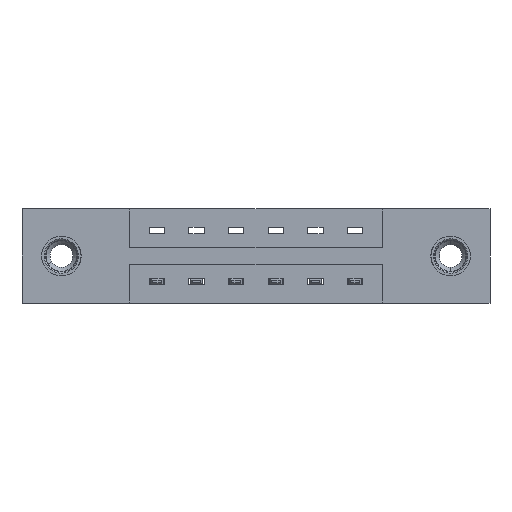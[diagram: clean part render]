
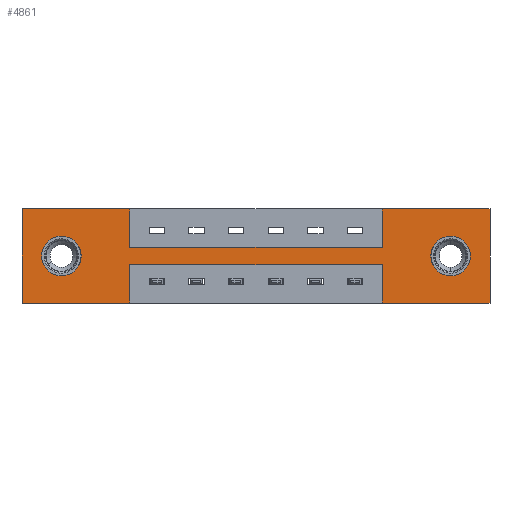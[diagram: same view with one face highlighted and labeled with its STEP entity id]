
A CAD part, front view. The second image highlights one B-rep face of the part: STEP entity #4861.
In plain terms, the highlighted planar face has unit normal (0, -1, 0).
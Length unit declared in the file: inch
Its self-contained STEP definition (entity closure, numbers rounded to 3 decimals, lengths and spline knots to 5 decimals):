
#3 = CARTESIAN_POINT ( 'NONE',  ( 1.417, 0., 0. ) ) ;
#84 = DIRECTION ( 'NONE',  ( 0., 1., 0. ) ) ;
#86 = CARTESIAN_POINT ( 'NONE',  ( 0., 0., -0.37 ) ) ;
#117 = VERTEX_POINT ( 'NONE', #8231 ) ;
#158 = EDGE_CURVE ( 'NONE', #1358, #7796, #9642, .T. ) ;
#309 = CARTESIAN_POINT ( 'NONE',  ( 0.155, 0., -0.185 ) ) ;
#356 = AXIS2_PLACEMENT_3D ( 'NONE', #9466, #7812, #4768 ) ;
#578 = ORIENTED_EDGE ( 'NONE', *, *, #1688, .F. ) ;
#599 = EDGE_LOOP ( 'NONE', ( #6540, #2924 ) ) ;
#604 = EDGE_CURVE ( 'NONE', #5155, #1770, #6991, .T. ) ;
#765 = EDGE_CURVE ( 'NONE', #10042, #5155, #3315, .T. ) ;
#847 = CARTESIAN_POINT ( 'NONE',  ( 0.425, 0., -0.22 ) ) ;
#882 = ORIENTED_EDGE ( 'NONE', *, *, #9879, .T. ) ;
#915 = VERTEX_POINT ( 'NONE', #2943 ) ;
#984 = ORIENTED_EDGE ( 'NONE', *, *, #6231, .T. ) ;
#1147 = CARTESIAN_POINT ( 'NONE',  ( 0.425, 0., 0. ) ) ;
#1316 = ORIENTED_EDGE ( 'NONE', *, *, #3263, .F. ) ;
#1358 = VERTEX_POINT ( 'NONE', #2992 ) ;
#1425 = CARTESIAN_POINT ( 'NONE',  ( 0., 0., -0.37 ) ) ;
#1584 = ORIENTED_EDGE ( 'NONE', *, *, #7878, .F. ) ;
#1679 = VECTOR ( 'NONE', #5977, 39.37008 ) ;
#1688 = EDGE_CURVE ( 'NONE', #4008, #117, #4629, .T. ) ;
#1770 = VERTEX_POINT ( 'NONE', #3680 ) ;
#1782 = VERTEX_POINT ( 'NONE', #7600 ) ;
#1876 = FACE_OUTER_BOUND ( 'NONE', #7864, .T. ) ;
#1889 = VERTEX_POINT ( 'NONE', #1425 ) ;
#1912 = CARTESIAN_POINT ( 'NONE',  ( 0., 0., 0. ) ) ;
#1924 = DIRECTION ( 'NONE',  ( 1., 0., 0. ) ) ;
#1983 = DIRECTION ( 'NONE',  ( 0., 0., -1. ) ) ;
#2023 = LINE ( 'NONE', #4361, #3880 ) ;
#2325 = PLANE ( 'NONE',  #356 ) ;
#2485 = DIRECTION ( 'NONE',  ( 0., 0., 1. ) ) ;
#2545 = VECTOR ( 'NONE', #1983, 39.37008 ) ;
#2671 = CARTESIAN_POINT ( 'NONE',  ( 1.687, 0., -0.263 ) ) ;
#2788 = CARTESIAN_POINT ( 'NONE',  ( 1.417, 0., -0.37 ) ) ;
#2924 = ORIENTED_EDGE ( 'NONE', *, *, #3849, .T. ) ;
#2937 = DIRECTION ( 'NONE',  ( 0., 0., -1. ) ) ;
#2943 = CARTESIAN_POINT ( 'NONE',  ( 0.425, 0., -0.37 ) ) ;
#2992 = CARTESIAN_POINT ( 'NONE',  ( 1.417, 0., -0.22 ) ) ;
#3064 = EDGE_CURVE ( 'NONE', #1770, #5269, #2023, .T. ) ;
#3070 = LINE ( 'NONE', #1912, #3682 ) ;
#3109 = AXIS2_PLACEMENT_3D ( 'NONE', #309, #8178, #6662 ) ;
#3122 = CIRCLE ( 'NONE', #3109, 0.078 ) ;
#3217 = AXIS2_PLACEMENT_3D ( 'NONE', #4790, #84, #6390 ) ;
#3255 = CARTESIAN_POINT ( 'NONE',  ( 0.155, 0., -0.185 ) ) ;
#3263 = EDGE_CURVE ( 'NONE', #7796, #915, #5581, .T. ) ;
#3315 = LINE ( 'NONE', #3959, #8549 ) ;
#3343 = AXIS2_PLACEMENT_3D ( 'NONE', #3255, #8640, #2485 ) ;
#3445 = CIRCLE ( 'NONE', #3989, 0.078 ) ;
#3448 = ORIENTED_EDGE ( 'NONE', *, *, #3064, .F. ) ;
#3455 = EDGE_LOOP ( 'NONE', ( #882, #984 ) ) ;
#3488 = DIRECTION ( 'NONE',  ( -1., 0., 0. ) ) ;
#3560 = VERTEX_POINT ( 'NONE', #8334 ) ;
#3680 = CARTESIAN_POINT ( 'NONE',  ( 1.417, 0., -0.15 ) ) ;
#3682 = VECTOR ( 'NONE', #9717, 39.37008 ) ;
#3849 = EDGE_CURVE ( 'NONE', #7292, #8692, #3122, .T. ) ;
#3880 = VECTOR ( 'NONE', #9771, 39.37008 ) ;
#3893 = CIRCLE ( 'NONE', #3343, 0.078 ) ;
#3951 = EDGE_CURVE ( 'NONE', #117, #5256, #4829, .T. ) ;
#3959 = CARTESIAN_POINT ( 'NONE',  ( 0.425, 0., 0. ) ) ;
#3989 = AXIS2_PLACEMENT_3D ( 'NONE', #5318, #9934, #2937 ) ;
#4008 = VERTEX_POINT ( 'NONE', #4646 ) ;
#4256 = LINE ( 'NONE', #86, #7430 ) ;
#4361 = CARTESIAN_POINT ( 'NONE',  ( 1.417, 0., 0. ) ) ;
#4436 = VECTOR ( 'NONE', #6579, 39.37008 ) ;
#4489 = DIRECTION ( 'NONE',  ( -1., 0., 0. ) ) ;
#4629 = LINE ( 'NONE', #8984, #2545 ) ;
#4646 = CARTESIAN_POINT ( 'NONE',  ( 1.842, 0., 0. ) ) ;
#4768 = DIRECTION ( 'NONE',  ( 0., 0., -1. ) ) ;
#4790 = CARTESIAN_POINT ( 'NONE',  ( 1.687, 0., -0.185 ) ) ;
#4829 = LINE ( 'NONE', #5167, #6813 ) ;
#4861 = ADVANCED_FACE ( 'NONE', ( #9311, #7987, #1876 ), #2325, .T. ) ;
#4890 = VECTOR ( 'NONE', #1924, 39.37008 ) ;
#4963 = CIRCLE ( 'NONE', #3217, 0.078 ) ;
#5005 = VECTOR ( 'NONE', #8905, 39.37008 ) ;
#5155 = VERTEX_POINT ( 'NONE', #9995 ) ;
#5167 = CARTESIAN_POINT ( 'NONE',  ( 0., 0., -0.37 ) ) ;
#5256 = VERTEX_POINT ( 'NONE', #9375 ) ;
#5269 = VERTEX_POINT ( 'NONE', #3 ) ;
#5318 = CARTESIAN_POINT ( 'NONE',  ( 1.687, 0., -0.185 ) ) ;
#5426 = EDGE_CURVE ( 'NONE', #3560, #10042, #9653, .T. ) ;
#5581 = LINE ( 'NONE', #9514, #9229 ) ;
#5663 = ORIENTED_EDGE ( 'NONE', *, *, #158, .F. ) ;
#5696 = DIRECTION ( 'NONE',  ( -1., 0., 0. ) ) ;
#5765 = VECTOR ( 'NONE', #3488, 39.37008 ) ;
#5977 = DIRECTION ( 'NONE',  ( 0., 0., 1. ) ) ;
#6231 = EDGE_CURVE ( 'NONE', #9949, #1782, #3445, .T. ) ;
#6390 = DIRECTION ( 'NONE',  ( 0., 0., -1. ) ) ;
#6540 = ORIENTED_EDGE ( 'NONE', *, *, #8009, .T. ) ;
#6579 = DIRECTION ( 'NONE',  ( 1., 0., 0. ) ) ;
#6589 = ORIENTED_EDGE ( 'NONE', *, *, #3951, .F. ) ;
#6662 = DIRECTION ( 'NONE',  ( 0., 0., 1. ) ) ;
#6813 = VECTOR ( 'NONE', #4489, 39.37008 ) ;
#6839 = EDGE_CURVE ( 'NONE', #1889, #3560, #3070, .T. ) ;
#6991 = LINE ( 'NONE', #8286, #4890 ) ;
#7097 = LINE ( 'NONE', #9666, #5005 ) ;
#7292 = VERTEX_POINT ( 'NONE', #7449 ) ;
#7327 = ORIENTED_EDGE ( 'NONE', *, *, #765, .F. ) ;
#7328 = EDGE_CURVE ( 'NONE', #5256, #1358, #8786, .T. ) ;
#7430 = VECTOR ( 'NONE', #5696, 39.37008 ) ;
#7449 = CARTESIAN_POINT ( 'NONE',  ( 0.155, 0., -0.263 ) ) ;
#7472 = EDGE_CURVE ( 'NONE', #5269, #4008, #7097, .T. ) ;
#7535 = ORIENTED_EDGE ( 'NONE', *, *, #6839, .F. ) ;
#7600 = CARTESIAN_POINT ( 'NONE',  ( 1.687, 0., -0.107 ) ) ;
#7796 = VERTEX_POINT ( 'NONE', #847 ) ;
#7802 = DIRECTION ( 'NONE',  ( 0., 0., -1. ) ) ;
#7812 = DIRECTION ( 'NONE',  ( 0., -1., 0. ) ) ;
#7864 = EDGE_LOOP ( 'NONE', ( #1316, #5663, #7936, #6589, #578, #8953, #3448, #8566, #7327, #8059, #7535, #1584 ) ) ;
#7878 = EDGE_CURVE ( 'NONE', #915, #1889, #4256, .T. ) ;
#7936 = ORIENTED_EDGE ( 'NONE', *, *, #7328, .F. ) ;
#7987 = FACE_BOUND ( 'NONE', #599, .T. ) ;
#8009 = EDGE_CURVE ( 'NONE', #8692, #7292, #3893, .T. ) ;
#8059 = ORIENTED_EDGE ( 'NONE', *, *, #5426, .F. ) ;
#8178 = DIRECTION ( 'NONE',  ( 0., 1., 0. ) ) ;
#8200 = CARTESIAN_POINT ( 'NONE',  ( 0., 0., 0. ) ) ;
#8231 = CARTESIAN_POINT ( 'NONE',  ( 1.842, 0., -0.37 ) ) ;
#8286 = CARTESIAN_POINT ( 'NONE',  ( 0.425, 0., -0.15 ) ) ;
#8334 = CARTESIAN_POINT ( 'NONE',  ( 0., 0., 0. ) ) ;
#8549 = VECTOR ( 'NONE', #7802, 39.37008 ) ;
#8566 = ORIENTED_EDGE ( 'NONE', *, *, #604, .F. ) ;
#8640 = DIRECTION ( 'NONE',  ( 0., 1., 0. ) ) ;
#8692 = VERTEX_POINT ( 'NONE', #9582 ) ;
#8751 = DIRECTION ( 'NONE',  ( 0., 0., -1. ) ) ;
#8786 = LINE ( 'NONE', #2788, #1679 ) ;
#8905 = DIRECTION ( 'NONE',  ( 1., 0., 0. ) ) ;
#8953 = ORIENTED_EDGE ( 'NONE', *, *, #7472, .F. ) ;
#8984 = CARTESIAN_POINT ( 'NONE',  ( 1.842, 0., 0. ) ) ;
#8997 = CARTESIAN_POINT ( 'NONE',  ( 0.425, 0., -0.22 ) ) ;
#9229 = VECTOR ( 'NONE', #8751, 39.37008 ) ;
#9311 = FACE_BOUND ( 'NONE', #3455, .T. ) ;
#9375 = CARTESIAN_POINT ( 'NONE',  ( 1.417, 0., -0.37 ) ) ;
#9466 = CARTESIAN_POINT ( 'NONE',  ( 0., 0., -0.37 ) ) ;
#9514 = CARTESIAN_POINT ( 'NONE',  ( 0.425, 0., -0.37 ) ) ;
#9582 = CARTESIAN_POINT ( 'NONE',  ( 0.155, 0., -0.107 ) ) ;
#9642 = LINE ( 'NONE', #8997, #5765 ) ;
#9653 = LINE ( 'NONE', #8200, #4436 ) ;
#9666 = CARTESIAN_POINT ( 'NONE',  ( 0., 0., 0. ) ) ;
#9717 = DIRECTION ( 'NONE',  ( 0., 0., 1. ) ) ;
#9771 = DIRECTION ( 'NONE',  ( 0., 0., 1. ) ) ;
#9879 = EDGE_CURVE ( 'NONE', #1782, #9949, #4963, .T. ) ;
#9934 = DIRECTION ( 'NONE',  ( 0., 1., 0. ) ) ;
#9949 = VERTEX_POINT ( 'NONE', #2671 ) ;
#9995 = CARTESIAN_POINT ( 'NONE',  ( 0.425, 0., -0.15 ) ) ;
#10042 = VERTEX_POINT ( 'NONE', #1147 ) ;
